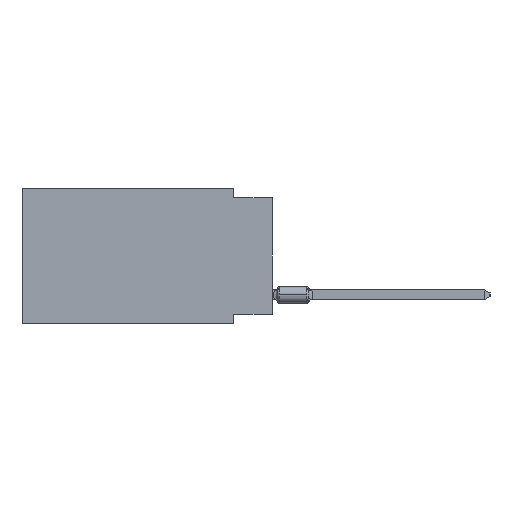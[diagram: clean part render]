
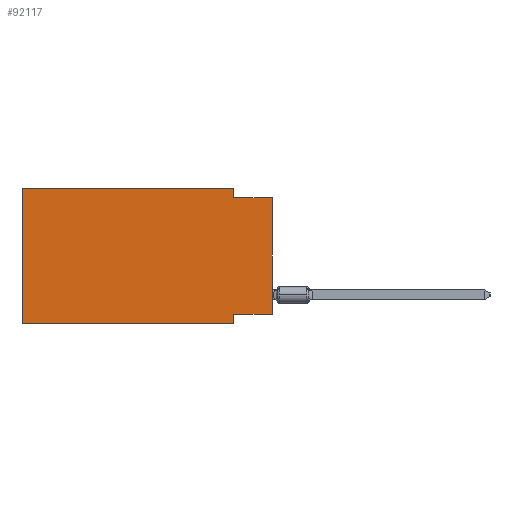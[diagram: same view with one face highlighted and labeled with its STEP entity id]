
A CAD part, left-side view. The second image highlights one B-rep face of the part: STEP entity #92117.
In plain terms, the highlighted planar face has unit normal (-1, 0, 0).
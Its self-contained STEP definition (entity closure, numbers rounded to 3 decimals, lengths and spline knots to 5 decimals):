
#654 = VERTEX_POINT ( 'NONE', #25760 ) ;
#2466 = CARTESIAN_POINT ( 'NONE',  ( 0., 0.645, 0. ) ) ;
#3020 = EDGE_CURVE ( 'NONE', #61415, #12233, #92937, .T. ) ;
#7867 = ORIENTED_EDGE ( 'NONE', *, *, #92656, .F. ) ;
#8331 = EDGE_CURVE ( 'NONE', #654, #95280, #82722, .T. ) ;
#10633 = CARTESIAN_POINT ( 'NONE',  ( 0., 0., -0.325 ) ) ;
#12233 = VERTEX_POINT ( 'NONE', #2466 ) ;
#12309 = EDGE_CURVE ( 'NONE', #12233, #71590, #78654, .T. ) ;
#12650 = VECTOR ( 'NONE', #113508, 39.37008 ) ;
#20415 = VERTEX_POINT ( 'NONE', #88801 ) ;
#20707 = CARTESIAN_POINT ( 'NONE',  ( 0., 0., -0.025 ) ) ;
#21223 = CARTESIAN_POINT ( 'NONE',  ( 0., 0., -0.025 ) ) ;
#22868 = VERTEX_POINT ( 'NONE', #42572 ) ;
#25267 = FACE_OUTER_BOUND ( 'NONE', #57022, .T. ) ;
#25760 = CARTESIAN_POINT ( 'NONE',  ( 0., 0., -0.325 ) ) ;
#26878 = CARTESIAN_POINT ( 'NONE',  ( 0., 0.645, -0.35 ) ) ;
#26881 = LINE ( 'NONE', #20707, #102342 ) ;
#34599 = EDGE_CURVE ( 'NONE', #61415, #20415, #91803, .T. ) ;
#38276 = VECTOR ( 'NONE', #71272, 39.37008 ) ;
#39467 = CARTESIAN_POINT ( 'NONE',  ( 0., 0.1, -0.325 ) ) ;
#41107 = DIRECTION ( 'NONE',  ( 0., -1., 0. ) ) ;
#41963 = DIRECTION ( 'NONE',  ( 0., 0., -1. ) ) ;
#42318 = CARTESIAN_POINT ( 'NONE',  ( 0., 0.645, 0. ) ) ;
#42572 = CARTESIAN_POINT ( 'NONE',  ( 0., 0.1, -0.025 ) ) ;
#44211 = AXIS2_PLACEMENT_3D ( 'NONE', #105681, #60396, #41963 ) ;
#44756 = DIRECTION ( 'NONE',  ( 0., -1., 0. ) ) ;
#45374 = VECTOR ( 'NONE', #54649, 39.37008 ) ;
#50014 = ORIENTED_EDGE ( 'NONE', *, *, #8331, .F. ) ;
#54649 = DIRECTION ( 'NONE',  ( 0., 0., -1. ) ) ;
#55923 = DIRECTION ( 'NONE',  ( 0., 1., 0. ) ) ;
#56979 = VECTOR ( 'NONE', #55923, 39.37008 ) ;
#57022 = EDGE_LOOP ( 'NONE', ( #73451, #7867, #66377, #113597, #78893, #94877, #68231, #50014 ) ) ;
#58698 = LINE ( 'NONE', #95043, #12650 ) ;
#60396 = DIRECTION ( 'NONE',  ( 1., 0., 0. ) ) ;
#61415 = VERTEX_POINT ( 'NONE', #89599 ) ;
#63022 = LINE ( 'NONE', #99912, #45374 ) ;
#63214 = DIRECTION ( 'NONE',  ( 0., -1., 0. ) ) ;
#66377 = ORIENTED_EDGE ( 'NONE', *, *, #80602, .F. ) ;
#67339 = CARTESIAN_POINT ( 'NONE',  ( 0., 0.645, 0. ) ) ;
#68231 = ORIENTED_EDGE ( 'NONE', *, *, #112720, .F. ) ;
#71272 = DIRECTION ( 'NONE',  ( 0., 0., -1. ) ) ;
#71590 = VERTEX_POINT ( 'NONE', #105530 ) ;
#73451 = ORIENTED_EDGE ( 'NONE', *, *, #85742, .T. ) ;
#78654 = LINE ( 'NONE', #42318, #113558 ) ;
#78893 = ORIENTED_EDGE ( 'NONE', *, *, #3020, .F. ) ;
#79034 = CARTESIAN_POINT ( 'NONE',  ( 0., 0.1, -0.35 ) ) ;
#80602 = EDGE_CURVE ( 'NONE', #71590, #22868, #63022, .T. ) ;
#82722 = LINE ( 'NONE', #10633, #56979 ) ;
#85742 = EDGE_CURVE ( 'NONE', #654, #90400, #58698, .T. ) ;
#88801 = CARTESIAN_POINT ( 'NONE',  ( 0., 0.1, -0.35 ) ) ;
#88963 = PLANE ( 'NONE',  #44211 ) ;
#89129 = LINE ( 'NONE', #79034, #38276 ) ;
#89599 = CARTESIAN_POINT ( 'NONE',  ( 0., 0.645, -0.35 ) ) ;
#90400 = VERTEX_POINT ( 'NONE', #21223 ) ;
#91803 = LINE ( 'NONE', #26878, #97392 ) ;
#92117 = ADVANCED_FACE ( 'NONE', ( #25267 ), #88963, .F. ) ;
#92656 = EDGE_CURVE ( 'NONE', #22868, #90400, #26881, .T. ) ;
#92937 = LINE ( 'NONE', #67339, #106945 ) ;
#94877 = ORIENTED_EDGE ( 'NONE', *, *, #34599, .T. ) ;
#95043 = CARTESIAN_POINT ( 'NONE',  ( 0., 0., 0. ) ) ;
#95280 = VERTEX_POINT ( 'NONE', #39467 ) ;
#97392 = VECTOR ( 'NONE', #63214, 39.37008 ) ;
#99912 = CARTESIAN_POINT ( 'NONE',  ( 0., 0.1, 0. ) ) ;
#102342 = VECTOR ( 'NONE', #44756, 39.37008 ) ;
#103643 = DIRECTION ( 'NONE',  ( 0., 0., 1. ) ) ;
#105530 = CARTESIAN_POINT ( 'NONE',  ( 0., 0.1, 0. ) ) ;
#105681 = CARTESIAN_POINT ( 'NONE',  ( 0., 0.645, 0. ) ) ;
#106945 = VECTOR ( 'NONE', #103643, 39.37008 ) ;
#112720 = EDGE_CURVE ( 'NONE', #95280, #20415, #89129, .T. ) ;
#113508 = DIRECTION ( 'NONE',  ( 0., 0., 1. ) ) ;
#113558 = VECTOR ( 'NONE', #41107, 39.37008 ) ;
#113597 = ORIENTED_EDGE ( 'NONE', *, *, #12309, .F. ) ;
